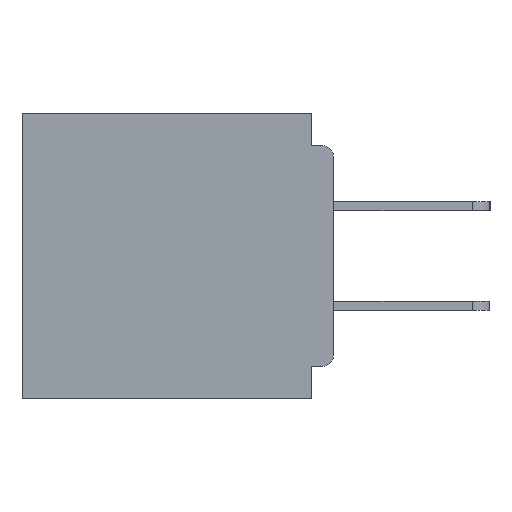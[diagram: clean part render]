
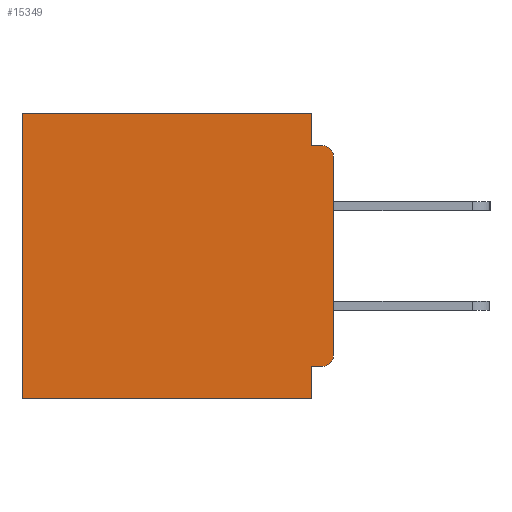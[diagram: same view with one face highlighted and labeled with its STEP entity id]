
A CAD part, left-side view. The second image highlights one B-rep face of the part: STEP entity #15349.
In plain terms, the highlighted planar face has unit normal (-1, 0, 0).
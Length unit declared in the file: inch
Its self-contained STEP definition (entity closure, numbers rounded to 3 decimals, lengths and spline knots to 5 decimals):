
#838 = VERTEX_POINT ( 'NONE', #10853 ) ;
#1004 = DIRECTION ( 'NONE',  ( 0., 0., -1. ) ) ;
#1154 = CARTESIAN_POINT ( 'NONE',  ( 0.3, 0., 0. ) ) ;
#1451 = CARTESIAN_POINT ( 'NONE',  ( 0.3, 0.031, 0. ) ) ;
#1718 = CARTESIAN_POINT ( 'NONE',  ( 0.3, 0.015, -0.355 ) ) ;
#1742 = VERTEX_POINT ( 'NONE', #1718 ) ;
#2065 = LINE ( 'NONE', #7631, #33716 ) ;
#2107 = VECTOR ( 'NONE', #32778, 39.37008 ) ;
#2157 = VECTOR ( 'NONE', #39079, 39.37008 ) ;
#2172 = VERTEX_POINT ( 'NONE', #9875 ) ;
#3558 = ORIENTED_EDGE ( 'NONE', *, *, #38731, .T. ) ;
#3664 = VERTEX_POINT ( 'NONE', #21943 ) ;
#4004 = VERTEX_POINT ( 'NONE', #40237 ) ;
#5122 = AXIS2_PLACEMENT_3D ( 'NONE', #38812, #19993, #1004 ) ;
#7249 = DIRECTION ( 'NONE',  ( 0., 1., 0. ) ) ;
#7250 = CARTESIAN_POINT ( 'NONE',  ( 0.3, 0., -0.06 ) ) ;
#7631 = CARTESIAN_POINT ( 'NONE',  ( 0.3, 0., -0.045 ) ) ;
#7708 = VERTEX_POINT ( 'NONE', #13993 ) ;
#7845 = DIRECTION ( 'NONE',  ( 0., 0., -1. ) ) ;
#8115 = CARTESIAN_POINT ( 'NONE',  ( 0.3, 0., -0.34 ) ) ;
#8320 = CARTESIAN_POINT ( 'NONE',  ( 0.3, 0.015, -0.06 ) ) ;
#9861 = CARTESIAN_POINT ( 'NONE',  ( 0.3, 0.031, -0.4 ) ) ;
#9875 = CARTESIAN_POINT ( 'NONE',  ( 0.3, 0.031, -0.4 ) ) ;
#9890 = EDGE_CURVE ( 'NONE', #32178, #13885, #23781, .T. ) ;
#10853 = CARTESIAN_POINT ( 'NONE',  ( 0.3, 0.437, -0.4 ) ) ;
#11501 = DIRECTION ( 'NONE',  ( 0., 0., -1. ) ) ;
#11673 = ORIENTED_EDGE ( 'NONE', *, *, #30321, .F. ) ;
#12266 = ORIENTED_EDGE ( 'NONE', *, *, #24806, .F. ) ;
#12452 = VECTOR ( 'NONE', #34793, 39.37008 ) ;
#13275 = EDGE_CURVE ( 'NONE', #4004, #838, #35732, .T. ) ;
#13885 = VERTEX_POINT ( 'NONE', #29435 ) ;
#13962 = DIRECTION ( 'NONE',  ( 0., -1., 0. ) ) ;
#13993 = CARTESIAN_POINT ( 'NONE',  ( 0.3, 0.031, -0.355 ) ) ;
#15289 = AXIS2_PLACEMENT_3D ( 'NONE', #8320, #30423, #11501 ) ;
#15347 = VECTOR ( 'NONE', #20998, 39.37008 ) ;
#15349 = ADVANCED_FACE ( 'NONE', ( #29290 ), #23616, .F. ) ;
#16190 = DIRECTION ( 'NONE',  ( 0., 0., -1. ) ) ;
#16768 = EDGE_CURVE ( 'NONE', #32178, #31707, #32141, .T. ) ;
#19915 = AXIS2_PLACEMENT_3D ( 'NONE', #39212, #26788, #7845 ) ;
#19993 = DIRECTION ( 'NONE',  ( -1., 0., 0. ) ) ;
#20017 = LINE ( 'NONE', #1154, #2157 ) ;
#20998 = DIRECTION ( 'NONE',  ( 0., 0., -1. ) ) ;
#21268 = ORIENTED_EDGE ( 'NONE', *, *, #28182, .F. ) ;
#21943 = CARTESIAN_POINT ( 'NONE',  ( 0.3, 0.031, -0.045 ) ) ;
#22732 = ORIENTED_EDGE ( 'NONE', *, *, #28941, .F. ) ;
#22889 = LINE ( 'NONE', #9861, #30257 ) ;
#23616 = PLANE ( 'NONE',  #19915 ) ;
#23781 = CIRCLE ( 'NONE', #15289, 0.015 ) ;
#24082 = CARTESIAN_POINT ( 'NONE',  ( 0.3, 0., -0.4 ) ) ;
#24373 = ORIENTED_EDGE ( 'NONE', *, *, #29718, .T. ) ;
#24806 = EDGE_CURVE ( 'NONE', #7708, #2172, #22889, .T. ) ;
#25150 = ORIENTED_EDGE ( 'NONE', *, *, #31097, .F. ) ;
#26056 = CARTESIAN_POINT ( 'NONE',  ( 0.3, 0., -0.4 ) ) ;
#26505 = EDGE_LOOP ( 'NONE', ( #38261, #34321, #21268, #25150, #3558, #38825, #11673, #12266, #22732, #24373 ) ) ;
#26788 = DIRECTION ( 'NONE',  ( 1., 0., 0. ) ) ;
#27392 = CARTESIAN_POINT ( 'NONE',  ( 0.3, 0.031, 0. ) ) ;
#28182 = EDGE_CURVE ( 'NONE', #3664, #13885, #2065, .T. ) ;
#28775 = CARTESIAN_POINT ( 'NONE',  ( 0.3, 0., -0.355 ) ) ;
#28941 = EDGE_CURVE ( 'NONE', #1742, #7708, #29243, .T. ) ;
#29243 = LINE ( 'NONE', #28775, #12452 ) ;
#29290 = FACE_OUTER_BOUND ( 'NONE', #26505, .T. ) ;
#29435 = CARTESIAN_POINT ( 'NONE',  ( 0.3, 0.015, -0.045 ) ) ;
#29490 = CARTESIAN_POINT ( 'NONE',  ( 0.3, 0.437, -0.4 ) ) ;
#29607 = VECTOR ( 'NONE', #29963, 39.37008 ) ;
#29718 = EDGE_CURVE ( 'NONE', #1742, #31707, #37019, .T. ) ;
#29963 = DIRECTION ( 'NONE',  ( 0., 0., -1. ) ) ;
#30257 = VECTOR ( 'NONE', #16190, 39.37008 ) ;
#30321 = EDGE_CURVE ( 'NONE', #2172, #838, #36462, .T. ) ;
#30423 = DIRECTION ( 'NONE',  ( -1., 0., 0. ) ) ;
#31097 = EDGE_CURVE ( 'NONE', #37078, #3664, #37918, .T. ) ;
#31707 = VERTEX_POINT ( 'NONE', #8115 ) ;
#32141 = LINE ( 'NONE', #24082, #15347 ) ;
#32178 = VERTEX_POINT ( 'NONE', #7250 ) ;
#32778 = DIRECTION ( 'NONE',  ( 0., 0., -1. ) ) ;
#33716 = VECTOR ( 'NONE', #13962, 39.37008 ) ;
#34321 = ORIENTED_EDGE ( 'NONE', *, *, #9890, .T. ) ;
#34508 = VECTOR ( 'NONE', #7249, 39.37008 ) ;
#34793 = DIRECTION ( 'NONE',  ( 0., 1., 0. ) ) ;
#35732 = LINE ( 'NONE', #29490, #2107 ) ;
#36462 = LINE ( 'NONE', #26056, #34508 ) ;
#37019 = CIRCLE ( 'NONE', #5122, 0.015 ) ;
#37078 = VERTEX_POINT ( 'NONE', #27392 ) ;
#37918 = LINE ( 'NONE', #1451, #29607 ) ;
#38261 = ORIENTED_EDGE ( 'NONE', *, *, #16768, .F. ) ;
#38731 = EDGE_CURVE ( 'NONE', #37078, #4004, #20017, .T. ) ;
#38812 = CARTESIAN_POINT ( 'NONE',  ( 0.3, 0.015, -0.34 ) ) ;
#38825 = ORIENTED_EDGE ( 'NONE', *, *, #13275, .T. ) ;
#39079 = DIRECTION ( 'NONE',  ( 0., 1., 0. ) ) ;
#39212 = CARTESIAN_POINT ( 'NONE',  ( 0.3, 0., -0.4 ) ) ;
#40237 = CARTESIAN_POINT ( 'NONE',  ( 0.3, 0.437, 0. ) ) ;
